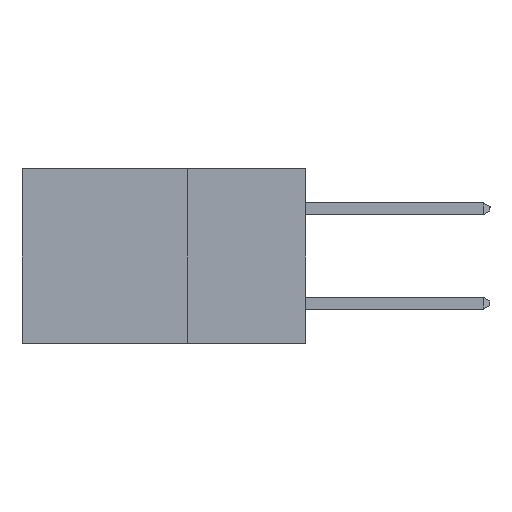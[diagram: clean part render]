
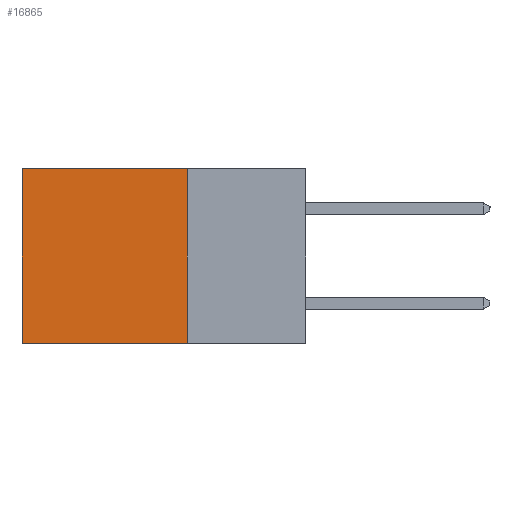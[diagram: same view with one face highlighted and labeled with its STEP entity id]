
A CAD part, left-side view. The second image highlights one B-rep face of the part: STEP entity #16865.
In plain terms, the highlighted planar face has unit normal (-1, 0, 0).
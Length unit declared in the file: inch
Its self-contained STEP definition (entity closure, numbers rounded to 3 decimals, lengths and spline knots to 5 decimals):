
#77 = VECTOR ( 'NONE', #7261, 39.37008 ) ;
#366 = VERTEX_POINT ( 'NONE', #4077 ) ;
#817 = EDGE_CURVE ( 'NONE', #24726, #22784, #8730, .T. ) ;
#2402 = ORIENTED_EDGE ( 'NONE', *, *, #817, .F. ) ;
#3148 = VECTOR ( 'NONE', #12959, 39.37008 ) ;
#3323 = PLANE ( 'NONE',  #25226 ) ;
#4077 = CARTESIAN_POINT ( 'NONE',  ( 0.2615, 0.25, 0. ) ) ;
#4142 = EDGE_LOOP ( 'NONE', ( #5247, #2402, #6975, #22075 ) ) ;
#4321 = EDGE_CURVE ( 'NONE', #366, #24726, #7898, .T. ) ;
#5247 = ORIENTED_EDGE ( 'NONE', *, *, #5533, .T. ) ;
#5533 = EDGE_CURVE ( 'NONE', #17343, #22784, #15407, .T. ) ;
#5622 = CARTESIAN_POINT ( 'NONE',  ( 0.2615, 0.25, 0. ) ) ;
#6975 = ORIENTED_EDGE ( 'NONE', *, *, #4321, .F. ) ;
#7261 = DIRECTION ( 'NONE',  ( 0., 0., -1. ) ) ;
#7644 = CARTESIAN_POINT ( 'NONE',  ( 0.2615, 0.25, -0.37 ) ) ;
#7898 = LINE ( 'NONE', #7644, #14342 ) ;
#8730 = LINE ( 'NONE', #16767, #3148 ) ;
#9009 = CARTESIAN_POINT ( 'NONE',  ( 0.2615, 0.25, -0.37 ) ) ;
#9624 = DIRECTION ( 'NONE',  ( 0., 0., -1. ) ) ;
#10652 = EDGE_CURVE ( 'NONE', #366, #17343, #15600, .T. ) ;
#11621 = FACE_OUTER_BOUND ( 'NONE', #4142, .T. ) ;
#12959 = DIRECTION ( 'NONE',  ( 0., 1., 0. ) ) ;
#13566 = DIRECTION ( 'NONE',  ( 0., 0., -1. ) ) ;
#13624 = DIRECTION ( 'NONE',  ( 0., 1., 0. ) ) ;
#14342 = VECTOR ( 'NONE', #9624, 39.37008 ) ;
#15281 = DIRECTION ( 'NONE',  ( 1., 0., 0. ) ) ;
#15407 = LINE ( 'NONE', #25182, #77 ) ;
#15600 = LINE ( 'NONE', #5622, #19117 ) ;
#16767 = CARTESIAN_POINT ( 'NONE',  ( 0.2615, 0.25, -0.37 ) ) ;
#16865 = ADVANCED_FACE ( 'NONE', ( #11621 ), #3323, .F. ) ;
#17343 = VERTEX_POINT ( 'NONE', #17625 ) ;
#17625 = CARTESIAN_POINT ( 'NONE',  ( 0.2615, 0.6, 0. ) ) ;
#19117 = VECTOR ( 'NONE', #13624, 39.37008 ) ;
#22075 = ORIENTED_EDGE ( 'NONE', *, *, #10652, .T. ) ;
#22784 = VERTEX_POINT ( 'NONE', #23117 ) ;
#23117 = CARTESIAN_POINT ( 'NONE',  ( 0.2615, 0.6, -0.37 ) ) ;
#24726 = VERTEX_POINT ( 'NONE', #9009 ) ;
#25182 = CARTESIAN_POINT ( 'NONE',  ( 0.2615, 0.6, -0.37 ) ) ;
#25226 = AXIS2_PLACEMENT_3D ( 'NONE', #25322, #15281, #13566 ) ;
#25322 = CARTESIAN_POINT ( 'NONE',  ( 0.2615, 0.25, -0.37 ) ) ;
